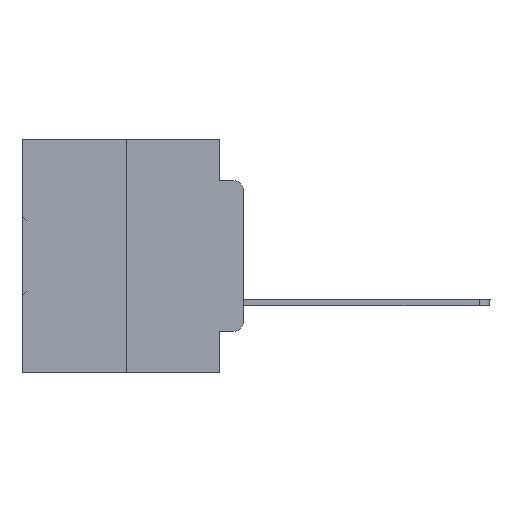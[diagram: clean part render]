
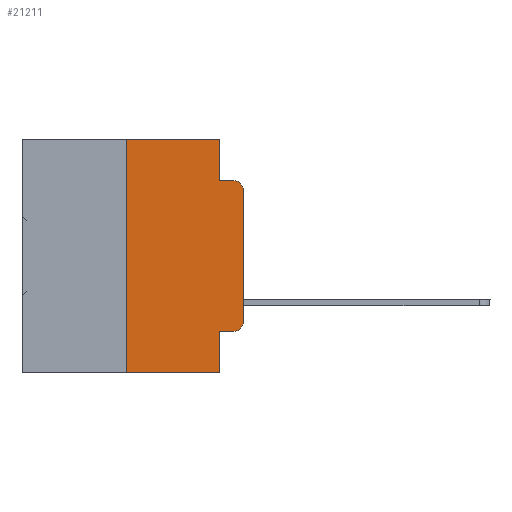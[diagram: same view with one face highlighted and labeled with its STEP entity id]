
A CAD part, left-side view. The second image highlights one B-rep face of the part: STEP entity #21211.
In plain terms, the highlighted planar face has unit normal (-1, 0, 0).
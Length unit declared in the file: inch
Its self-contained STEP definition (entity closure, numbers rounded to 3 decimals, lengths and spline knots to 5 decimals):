
#1428 = DIRECTION ( 'NONE',  ( 0., -1., 0. ) ) ;
#1903 = AXIS2_PLACEMENT_3D ( 'NONE', #27219, #18322, #13480 ) ;
#1978 = VERTEX_POINT ( 'NONE', #19338 ) ;
#2339 = CARTESIAN_POINT ( 'NONE',  ( 0., 0.051, -0.4115 ) ) ;
#2692 = DIRECTION ( 'NONE',  ( 0., -1., 0. ) ) ;
#3113 = VERTEX_POINT ( 'NONE', #12855 ) ;
#3303 = CARTESIAN_POINT ( 'NONE',  ( 0., 0.051, -0.5 ) ) ;
#3714 = PLANE ( 'NONE',  #4756 ) ;
#4073 = CARTESIAN_POINT ( 'NONE',  ( 0., 0.473, 0. ) ) ;
#4267 = EDGE_CURVE ( 'NONE', #27031, #3113, #5631, .T. ) ;
#4756 = AXIS2_PLACEMENT_3D ( 'NONE', #4073, #15397, #26711 ) ;
#4908 = CARTESIAN_POINT ( 'NONE',  ( 0., 0.051, 0. ) ) ;
#5631 = LINE ( 'NONE', #4908, #24084 ) ;
#5685 = EDGE_CURVE ( 'NONE', #21870, #27031, #25837, .T. ) ;
#5686 = VERTEX_POINT ( 'NONE', #29000 ) ;
#5745 = ORIENTED_EDGE ( 'NONE', *, *, #5685, .F. ) ;
#6371 = DIRECTION ( 'NONE',  ( 0., -1., 0. ) ) ;
#6501 = VERTEX_POINT ( 'NONE', #20559 ) ;
#8229 = ORIENTED_EDGE ( 'NONE', *, *, #16860, .T. ) ;
#9310 = EDGE_CURVE ( 'NONE', #5686, #12617, #32382, .T. ) ;
#9321 = ORIENTED_EDGE ( 'NONE', *, *, #21915, .F. ) ;
#9773 = EDGE_LOOP ( 'NONE', ( #8229, #35424, #32255, #21876, #5745, #9321, #10286, #15392, #13478, #14895 ) ) ;
#9899 = CARTESIAN_POINT ( 'NONE',  ( 0., 0.473, -0.5 ) ) ;
#10181 = LINE ( 'NONE', #21494, #21906 ) ;
#10286 = ORIENTED_EDGE ( 'NONE', *, *, #16748, .T. ) ;
#10651 = DIRECTION ( 'NONE',  ( 0., 0., -1. ) ) ;
#11727 = CARTESIAN_POINT ( 'NONE',  ( 0., 0.25, 0. ) ) ;
#12617 = VERTEX_POINT ( 'NONE', #29838 ) ;
#12822 = AXIS2_PLACEMENT_3D ( 'NONE', #33818, #36066, #31022 ) ;
#12855 = CARTESIAN_POINT ( 'NONE',  ( 0., 0.051, -0.0885 ) ) ;
#13478 = ORIENTED_EDGE ( 'NONE', *, *, #15698, .T. ) ;
#13480 = DIRECTION ( 'NONE',  ( 0., 0., -1. ) ) ;
#14131 = VECTOR ( 'NONE', #6371, 39.37008 ) ;
#14194 = LINE ( 'NONE', #2339, #30591 ) ;
#14340 = DIRECTION ( 'NONE',  ( 0., 0., 1. ) ) ;
#14895 = ORIENTED_EDGE ( 'NONE', *, *, #9310, .T. ) ;
#14916 = CIRCLE ( 'NONE', #1903, 0.02 ) ;
#15388 = DIRECTION ( 'NONE',  ( 0., 0., -1. ) ) ;
#15392 = ORIENTED_EDGE ( 'NONE', *, *, #34059, .F. ) ;
#15397 = DIRECTION ( 'NONE',  ( 1., 0., 0. ) ) ;
#15698 = EDGE_CURVE ( 'NONE', #17895, #5686, #14194, .T. ) ;
#16199 = DIRECTION ( 'NONE',  ( 0., 0., 1. ) ) ;
#16454 = CARTESIAN_POINT ( 'NONE',  ( 0., 0., -0.1085 ) ) ;
#16748 = EDGE_CURVE ( 'NONE', #6501, #31017, #18072, .T. ) ;
#16860 = EDGE_CURVE ( 'NONE', #12617, #23244, #32735, .T. ) ;
#16936 = CARTESIAN_POINT ( 'NONE',  ( 0., 0.051, 0. ) ) ;
#17133 = LINE ( 'NONE', #28442, #24351 ) ;
#17895 = VERTEX_POINT ( 'NONE', #26045 ) ;
#18072 = LINE ( 'NONE', #9899, #36501 ) ;
#18313 = LINE ( 'NONE', #35581, #21716 ) ;
#18322 = DIRECTION ( 'NONE',  ( -1., 0., 0. ) ) ;
#19338 = CARTESIAN_POINT ( 'NONE',  ( 0., 0.02, -0.0885 ) ) ;
#20559 = CARTESIAN_POINT ( 'NONE',  ( 0., 0.25, -0.5 ) ) ;
#21211 = ADVANCED_FACE ( 'NONE', ( #23373 ), #3714, .F. ) ;
#21494 = CARTESIAN_POINT ( 'NONE',  ( 0., 0.051, 0. ) ) ;
#21716 = VECTOR ( 'NONE', #1428, 39.37008 ) ;
#21870 = VERTEX_POINT ( 'NONE', #11727 ) ;
#21876 = ORIENTED_EDGE ( 'NONE', *, *, #4267, .F. ) ;
#21906 = VECTOR ( 'NONE', #15388, 39.37008 ) ;
#21915 = EDGE_CURVE ( 'NONE', #6501, #21870, #17133, .T. ) ;
#23077 = EDGE_CURVE ( 'NONE', #23244, #1978, #14916, .T. ) ;
#23244 = VERTEX_POINT ( 'NONE', #16454 ) ;
#23373 = FACE_OUTER_BOUND ( 'NONE', #9773, .T. ) ;
#24084 = VECTOR ( 'NONE', #10651, 39.37008 ) ;
#24351 = VECTOR ( 'NONE', #14340, 39.37008 ) ;
#25837 = LINE ( 'NONE', #26023, #14131 ) ;
#26023 = CARTESIAN_POINT ( 'NONE',  ( 0., 0.473, 0. ) ) ;
#26045 = CARTESIAN_POINT ( 'NONE',  ( 0., 0.051, -0.4115 ) ) ;
#26711 = DIRECTION ( 'NONE',  ( 0., 0., -1. ) ) ;
#27031 = VERTEX_POINT ( 'NONE', #16936 ) ;
#27219 = CARTESIAN_POINT ( 'NONE',  ( 0., 0.02, -0.1085 ) ) ;
#27333 = CARTESIAN_POINT ( 'NONE',  ( 0., 0., 0. ) ) ;
#28442 = CARTESIAN_POINT ( 'NONE',  ( 0., 0.25, 0. ) ) ;
#29000 = CARTESIAN_POINT ( 'NONE',  ( 0., 0.02, -0.4115 ) ) ;
#29368 = EDGE_CURVE ( 'NONE', #3113, #1978, #18313, .T. ) ;
#29385 = DIRECTION ( 'NONE',  ( 0., -1., 0. ) ) ;
#29838 = CARTESIAN_POINT ( 'NONE',  ( 0., 0., -0.3915 ) ) ;
#30591 = VECTOR ( 'NONE', #2692, 39.37008 ) ;
#31017 = VERTEX_POINT ( 'NONE', #3303 ) ;
#31022 = DIRECTION ( 'NONE',  ( 0., 0., -1. ) ) ;
#32255 = ORIENTED_EDGE ( 'NONE', *, *, #29368, .F. ) ;
#32382 = CIRCLE ( 'NONE', #12822, 0.02 ) ;
#32735 = LINE ( 'NONE', #27333, #36549 ) ;
#33818 = CARTESIAN_POINT ( 'NONE',  ( 0., 0.02, -0.3915 ) ) ;
#34059 = EDGE_CURVE ( 'NONE', #17895, #31017, #10181, .T. ) ;
#35424 = ORIENTED_EDGE ( 'NONE', *, *, #23077, .T. ) ;
#35581 = CARTESIAN_POINT ( 'NONE',  ( 0., 0.051, -0.0885 ) ) ;
#36066 = DIRECTION ( 'NONE',  ( -1., 0., 0. ) ) ;
#36501 = VECTOR ( 'NONE', #29385, 39.37008 ) ;
#36549 = VECTOR ( 'NONE', #16199, 39.37008 ) ;
